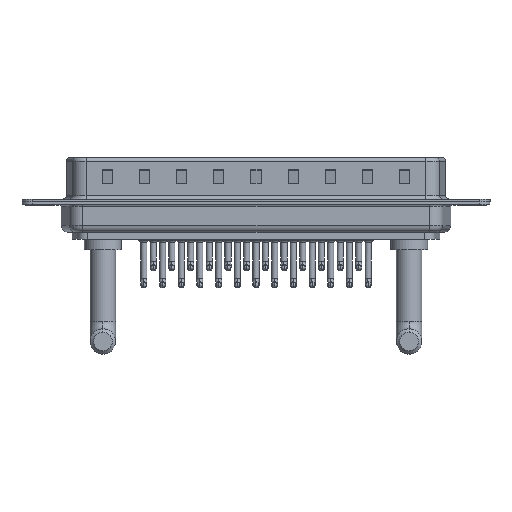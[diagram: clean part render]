
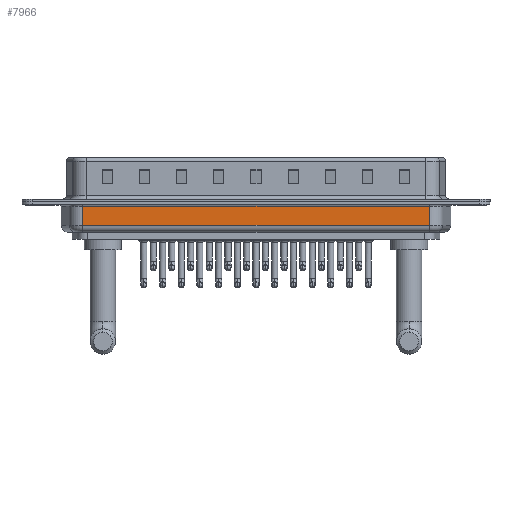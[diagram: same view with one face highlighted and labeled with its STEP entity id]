
A CAD part, front view. The second image highlights one B-rep face of the part: STEP entity #7966.
In plain terms, the highlighted planar face has unit normal (0, -1, 0).
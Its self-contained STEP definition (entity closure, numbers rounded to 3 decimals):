
#1460 = VECTOR ( 'NONE', #25928, 1000. ) ;
#1485 = CARTESIAN_POINT ( 'NONE',  ( 57.469, -5.35, -4.5 ) ) ;
#2036 = ORIENTED_EDGE ( 'NONE', *, *, #14045, .T. ) ;
#2642 = VERTEX_POINT ( 'NONE', #7833 ) ;
#2908 = PLANE ( 'NONE',  #23155 ) ;
#3925 = VERTEX_POINT ( 'NONE', #11903 ) ;
#4837 = ORIENTED_EDGE ( 'NONE', *, *, #23274, .T. ) ;
#4928 = VERTEX_POINT ( 'NONE', #21103 ) ;
#5801 = LINE ( 'NONE', #1485, #10970 ) ;
#6198 = DIRECTION ( 'NONE',  ( 1., 0., 0. ) ) ;
#7194 = ORIENTED_EDGE ( 'NONE', *, *, #15211, .T. ) ;
#7421 = VECTOR ( 'NONE', #8955, 1000. ) ;
#7833 = CARTESIAN_POINT ( 'NONE',  ( 57.469, -5.35, -0.65 ) ) ;
#7966 = ADVANCED_FACE ( 'NONE', ( #19394 ), #2908, .F. ) ;
#8603 = DIRECTION ( 'NONE',  ( -1., 0., 0. ) ) ;
#8955 = DIRECTION ( 'NONE',  ( 0., 0., 1. ) ) ;
#10394 = LINE ( 'NONE', #16471, #16490 ) ;
#10970 = VECTOR ( 'NONE', #18367, 1000. ) ;
#11903 = CARTESIAN_POINT ( 'NONE',  ( 6.031, -5.35, -0.65 ) ) ;
#12127 = EDGE_CURVE ( 'NONE', #4928, #3925, #25325, .T. ) ;
#13009 = CARTESIAN_POINT ( 'NONE',  ( 6.031, -5.35, -4.5 ) ) ;
#14045 = EDGE_CURVE ( 'NONE', #4928, #20171, #10394, .T. ) ;
#14993 = CARTESIAN_POINT ( 'NONE',  ( 57.469, -5.35, -3.5 ) ) ;
#15211 = EDGE_CURVE ( 'NONE', #2642, #3925, #19539, .T. ) ;
#16471 = CARTESIAN_POINT ( 'NONE',  ( 6.031, -5.35, -3.5 ) ) ;
#16490 = VECTOR ( 'NONE', #6198, 1000. ) ;
#18367 = DIRECTION ( 'NONE',  ( 0., 0., 1. ) ) ;
#18873 = CARTESIAN_POINT ( 'NONE',  ( 6.031, -5.35, -4.5 ) ) ;
#19394 = FACE_OUTER_BOUND ( 'NONE', #25278, .T. ) ;
#19539 = LINE ( 'NONE', #21848, #1460 ) ;
#20171 = VERTEX_POINT ( 'NONE', #14993 ) ;
#21103 = CARTESIAN_POINT ( 'NONE',  ( 6.031, -5.35, -3.5 ) ) ;
#21848 = CARTESIAN_POINT ( 'NONE',  ( 6.031, -5.35, -0.65 ) ) ;
#22471 = ORIENTED_EDGE ( 'NONE', *, *, #12127, .F. ) ;
#23155 = AXIS2_PLACEMENT_3D ( 'NONE', #18873, #23326, #8603 ) ;
#23274 = EDGE_CURVE ( 'NONE', #20171, #2642, #5801, .T. ) ;
#23326 = DIRECTION ( 'NONE',  ( 0., 1., 0. ) ) ;
#25278 = EDGE_LOOP ( 'NONE', ( #22471, #2036, #4837, #7194 ) ) ;
#25325 = LINE ( 'NONE', #13009, #7421 ) ;
#25928 = DIRECTION ( 'NONE',  ( -1., 0., 0. ) ) ;
